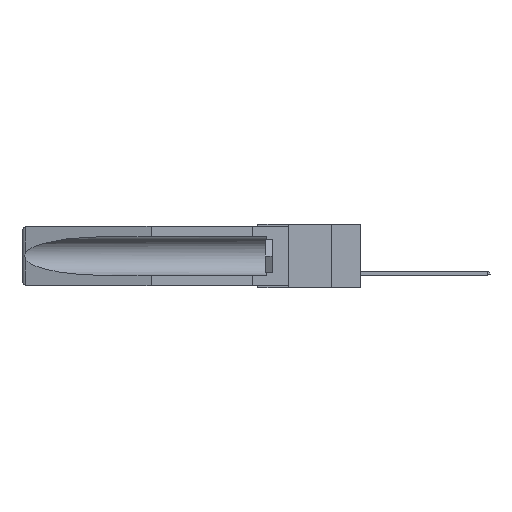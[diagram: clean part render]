
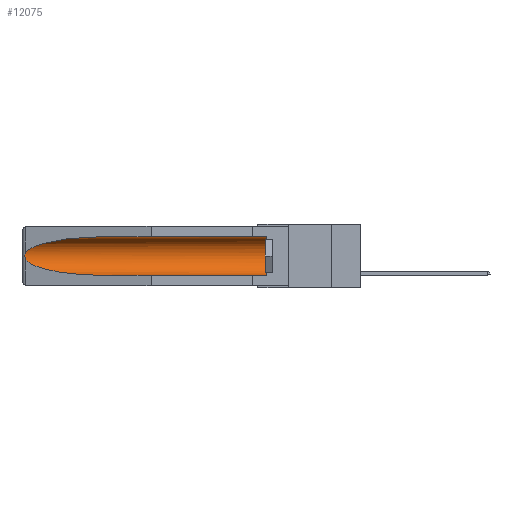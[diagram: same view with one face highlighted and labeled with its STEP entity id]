
A CAD part, left-side view. The second image highlights one B-rep face of the part: STEP entity #12075.
In plain terms, the highlighted cylindrical face has radius 2.857 mm (diameter 5.715 mm), a partial arc.
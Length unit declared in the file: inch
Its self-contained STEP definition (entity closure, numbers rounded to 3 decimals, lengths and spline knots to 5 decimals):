
#745 = CARTESIAN_POINT ( 'NONE',  ( 0.21114, 1.30732, -0.284 ) ) ;
#837 = CARTESIAN_POINT ( 'NONE',  ( 0.26654, 1.53092, -0.15636 ) ) ;
#951 = VECTOR ( 'NONE', #25778, 39.37008 ) ;
#1266 = CARTESIAN_POINT ( 'NONE',  ( 0.26537, 1.52718, -0.14972 ) ) ;
#2115 = FACE_OUTER_BOUND ( 'NONE', #15875, .T. ) ;
#2348 = EDGE_CURVE ( 'NONE', #12519, #17534, #26172, .T. ) ;
#3448 = CARTESIAN_POINT ( 'NONE',  ( 0.25451, 1.48313, -0.09465 ) ) ;
#4043 = ORIENTED_EDGE ( 'NONE', *, *, #2348, .T. ) ;
#4419 = ORIENTED_EDGE ( 'NONE', *, *, #10926, .T. ) ;
#4581 = DIRECTION ( 'NONE',  ( 0., 0., 1. ) ) ;
#5626 = CARTESIAN_POINT ( 'NONE',  ( 0.26537, 1.52718, -0.19328 ) ) ;
#5862 = VERTEX_POINT ( 'NONE', #21448 ) ;
#6186 = ORIENTED_EDGE ( 'NONE', *, *, #20824, .T. ) ;
#6819 = CYLINDRICAL_SURFACE ( 'NONE', #23086, 0.1125 ) ;
#7000 = CARTESIAN_POINT ( 'NONE',  ( 0.26537, 1.52718, -0.14972 ) ) ;
#7095 = CARTESIAN_POINT ( 'NONE',  ( 0.155, -0.30754, -0.284 ) ) ;
#7205 = DIRECTION ( 'NONE',  ( 0., 1., 0. ) ) ;
#7351 = DIRECTION ( 'NONE',  ( 0., 0., 1. ) ) ;
#8187 =( BOUNDED_CURVE ( )  B_SPLINE_CURVE ( 3, ( #14708, #28713, #745, #26326 ),
 .UNSPECIFIED., .F., .T. ) 
 B_SPLINE_CURVE_WITH_KNOTS ( ( 4, 4 ),
 ( 0.1948, 1.5708 ),
 .UNSPECIFIED. ) 
 CURVE ( )  GEOMETRIC_REPRESENTATION_ITEM ( )  RATIONAL_B_SPLINE_CURVE ( ( 1., 0.848, 0.848, 1. ) ) 
 REPRESENTATION_ITEM ( '' )  );
#8350 = CARTESIAN_POINT ( 'NONE',  ( 0.155, 1.07973, -0.059 ) ) ;
#10356 = CARTESIAN_POINT ( 'NONE',  ( 0.26537, 1.52718, -0.14972 ) ) ;
#10808 = ORIENTED_EDGE ( 'NONE', *, *, #12529, .F. ) ;
#10926 = EDGE_CURVE ( 'NONE', #17534, #5862, #8187, .T. ) ;
#11981 = CARTESIAN_POINT ( 'NONE',  ( 0.155, -0.30754, -0.1715 ) ) ;
#12075 = ADVANCED_FACE ( 'NONE', ( #2115 ), #6819, .F. ) ;
#12453 = CARTESIAN_POINT ( 'NONE',  ( 0.26655, 1.53094, -0.18657 ) ) ;
#12465 = EDGE_CURVE ( 'NONE', #24800, #12519, #25287, .T. ) ;
#12519 = VERTEX_POINT ( 'NONE', #7000 ) ;
#12529 = EDGE_CURVE ( 'NONE', #14771, #5862, #27700, .T. ) ;
#14708 = CARTESIAN_POINT ( 'NONE',  ( 0.26537, 1.52718, -0.19328 ) ) ;
#14771 = VERTEX_POINT ( 'NONE', #18955 ) ;
#14798 = CARTESIAN_POINT ( 'NONE',  ( 0.26597, 1.5296, -0.19026 ) ) ;
#15875 = EDGE_LOOP ( 'NONE', ( #22761, #4043, #4419, #10808, #16769, #6186 ) ) ;
#16769 = ORIENTED_EDGE ( 'NONE', *, *, #18964, .T. ) ;
#16995 = CARTESIAN_POINT ( 'NONE',  ( 0.2675, 1.53308, -0.16763 ) ) ;
#17534 = VERTEX_POINT ( 'NONE', #26144 ) ;
#17540 = CARTESIAN_POINT ( 'NONE',  ( 0.21114, 1.30732, -0.059 ) ) ;
#18376 = DIRECTION ( 'NONE',  ( 0., -1., 0. ) ) ;
#18955 = CARTESIAN_POINT ( 'NONE',  ( 0.155, 0.126, -0.284 ) ) ;
#18964 = EDGE_CURVE ( 'NONE', #14771, #21056, #20080, .T. ) ;
#19907 = AXIS2_PLACEMENT_3D ( 'NONE', #27668, #18376, #4581 ) ;
#20080 = CIRCLE ( 'NONE', #19907, 0.1125 ) ;
#20824 = EDGE_CURVE ( 'NONE', #21056, #24800, #29381, .T. ) ;
#21056 = VERTEX_POINT ( 'NONE', #29669 ) ;
#21371 = DIRECTION ( 'NONE',  ( 0., 1., 0. ) ) ;
#21448 = CARTESIAN_POINT ( 'NONE',  ( 0.155, 1.07973, -0.284 ) ) ;
#21665 = CARTESIAN_POINT ( 'NONE',  ( 0.2675, 1.53308, -0.17534 ) ) ;
#22153 = CARTESIAN_POINT ( 'NONE',  ( 0.155, 1.07973, -0.059 ) ) ;
#22761 = ORIENTED_EDGE ( 'NONE', *, *, #12465, .T. ) ;
#23086 = AXIS2_PLACEMENT_3D ( 'NONE', #11981, #21371, #7351 ) ;
#23895 = CARTESIAN_POINT ( 'NONE',  ( 0.26597, 1.52961, -0.15275 ) ) ;
#24800 = VERTEX_POINT ( 'NONE', #22153 ) ;
#25287 =( BOUNDED_CURVE ( )  B_SPLINE_CURVE ( 3, ( #8350, #17540, #3448, #10356 ),
 .UNSPECIFIED., .F., .F. ) 
 B_SPLINE_CURVE_WITH_KNOTS ( ( 4, 4 ),
 ( 4.71239, 6.08839 ),
 .UNSPECIFIED. ) 
 CURVE ( )  GEOMETRIC_REPRESENTATION_ITEM ( )  RATIONAL_B_SPLINE_CURVE ( ( 1., 0.848, 0.848, 1. ) ) 
 REPRESENTATION_ITEM ( '' )  );
#25778 = DIRECTION ( 'NONE',  ( 0., 1., 0. ) ) ;
#26144 = CARTESIAN_POINT ( 'NONE',  ( 0.26537, 1.52718, -0.19328 ) ) ;
#26172 = B_SPLINE_CURVE_WITH_KNOTS ( 'NONE', 3,
 ( #1266, #23895, #837, #26423, #16995, #21665, #26322, #12453, #14798, #5626 ),
 .UNSPECIFIED., .F., .F.,
 ( 4, 2, 2, 2, 4 ),
 ( 0., 0.00029, 0.00058, 0.00087, 0.00117 ),
 .UNSPECIFIED. ) ;
#26322 = CARTESIAN_POINT ( 'NONE',  ( 0.2673, 1.53269, -0.17917 ) ) ;
#26326 = CARTESIAN_POINT ( 'NONE',  ( 0.155, 1.07973, -0.284 ) ) ;
#26423 = CARTESIAN_POINT ( 'NONE',  ( 0.2673, 1.5327, -0.16383 ) ) ;
#27668 = CARTESIAN_POINT ( 'NONE',  ( 0.155, 0.126, -0.1715 ) ) ;
#27700 = LINE ( 'NONE', #7095, #951 ) ;
#27783 = CARTESIAN_POINT ( 'NONE',  ( 0.155, -0.30754, -0.059 ) ) ;
#28653 = VECTOR ( 'NONE', #7205, 39.37008 ) ;
#28713 = CARTESIAN_POINT ( 'NONE',  ( 0.25451, 1.48313, -0.24835 ) ) ;
#29381 = LINE ( 'NONE', #27783, #28653 ) ;
#29669 = CARTESIAN_POINT ( 'NONE',  ( 0.155, 0.126, -0.059 ) ) ;
